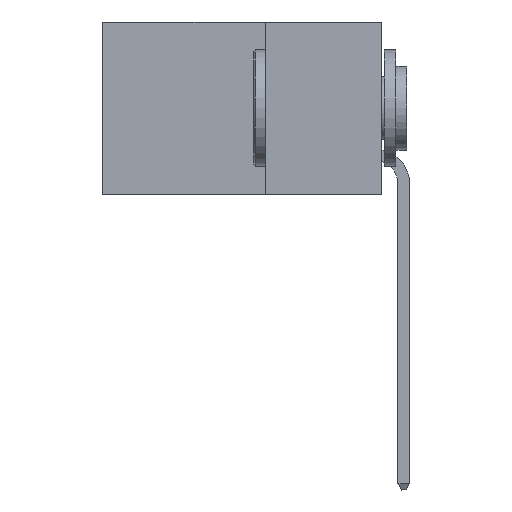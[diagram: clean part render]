
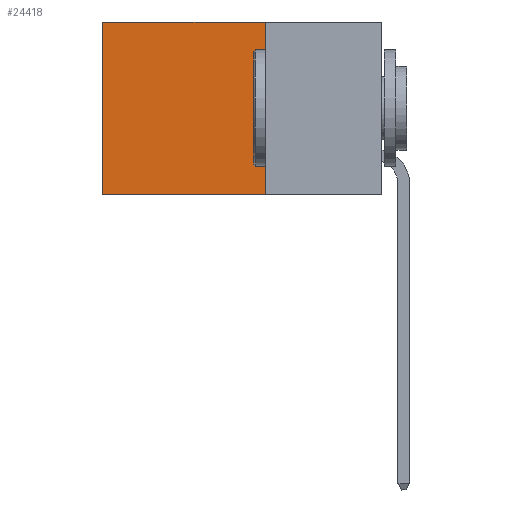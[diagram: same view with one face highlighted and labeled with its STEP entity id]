
A CAD part, left-side view. The second image highlights one B-rep face of the part: STEP entity #24418.
In plain terms, the highlighted planar face has unit normal (-1, 0, 0).
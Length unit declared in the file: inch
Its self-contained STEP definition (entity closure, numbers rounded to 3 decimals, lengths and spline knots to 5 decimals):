
#102 = ORIENTED_EDGE ( 'NONE', *, *, #18180, .F. ) ;
#238 = PLANE ( 'NONE',  #28775 ) ;
#312 = CARTESIAN_POINT ( 'NONE',  ( 0.2875, 0.25, 0. ) ) ;
#861 = VERTEX_POINT ( 'NONE', #30750 ) ;
#1405 = FACE_OUTER_BOUND ( 'NONE', #2825, .T. ) ;
#2391 = CARTESIAN_POINT ( 'NONE',  ( 0.2875, 0.25, -0.37 ) ) ;
#2825 = EDGE_LOOP ( 'NONE', ( #28382, #102, #34598, #34795 ) ) ;
#8444 = LINE ( 'NONE', #31611, #15999 ) ;
#11381 = EDGE_CURVE ( 'NONE', #27991, #861, #17231, .T. ) ;
#11905 = CARTESIAN_POINT ( 'NONE',  ( 0.2875, 0.6, 0. ) ) ;
#13298 = DIRECTION ( 'NONE',  ( 0., 1., 0. ) ) ;
#13398 = DIRECTION ( 'NONE',  ( 1., 0., 0. ) ) ;
#15399 = DIRECTION ( 'NONE',  ( 0., 1., 0. ) ) ;
#15999 = VECTOR ( 'NONE', #15399, 39.37008 ) ;
#17031 = LINE ( 'NONE', #312, #27552 ) ;
#17231 = LINE ( 'NONE', #11905, #22727 ) ;
#18180 = EDGE_CURVE ( 'NONE', #19732, #861, #18594, .T. ) ;
#18209 = DIRECTION ( 'NONE',  ( 0., 0., -1. ) ) ;
#18594 = LINE ( 'NONE', #35521, #40634 ) ;
#19310 = CARTESIAN_POINT ( 'NONE',  ( 0.2875, 0.25, 0. ) ) ;
#19732 = VERTEX_POINT ( 'NONE', #2391 ) ;
#20832 = EDGE_CURVE ( 'NONE', #23290, #27991, #8444, .T. ) ;
#22727 = VECTOR ( 'NONE', #18209, 39.37008 ) ;
#22797 = DIRECTION ( 'NONE',  ( 0., 0., -1. ) ) ;
#23290 = VERTEX_POINT ( 'NONE', #36133 ) ;
#24418 = ADVANCED_FACE ( 'NONE', ( #1405 ), #238, .F. ) ;
#27552 = VECTOR ( 'NONE', #39332, 39.37008 ) ;
#27991 = VERTEX_POINT ( 'NONE', #31058 ) ;
#28382 = ORIENTED_EDGE ( 'NONE', *, *, #11381, .T. ) ;
#28775 = AXIS2_PLACEMENT_3D ( 'NONE', #19310, #13398, #22797 ) ;
#30750 = CARTESIAN_POINT ( 'NONE',  ( 0.2875, 0.6, -0.37 ) ) ;
#31058 = CARTESIAN_POINT ( 'NONE',  ( 0.2875, 0.6, 0. ) ) ;
#31611 = CARTESIAN_POINT ( 'NONE',  ( 0.2875, 0.25, 0. ) ) ;
#34598 = ORIENTED_EDGE ( 'NONE', *, *, #40609, .F. ) ;
#34795 = ORIENTED_EDGE ( 'NONE', *, *, #20832, .T. ) ;
#35521 = CARTESIAN_POINT ( 'NONE',  ( 0.2875, 0.25, -0.37 ) ) ;
#36133 = CARTESIAN_POINT ( 'NONE',  ( 0.2875, 0.25, 0. ) ) ;
#39332 = DIRECTION ( 'NONE',  ( 0., 0., -1. ) ) ;
#40609 = EDGE_CURVE ( 'NONE', #23290, #19732, #17031, .T. ) ;
#40634 = VECTOR ( 'NONE', #13298, 39.37008 ) ;
